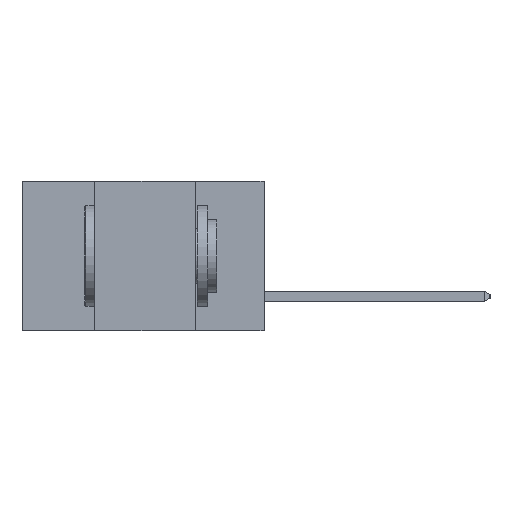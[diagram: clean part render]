
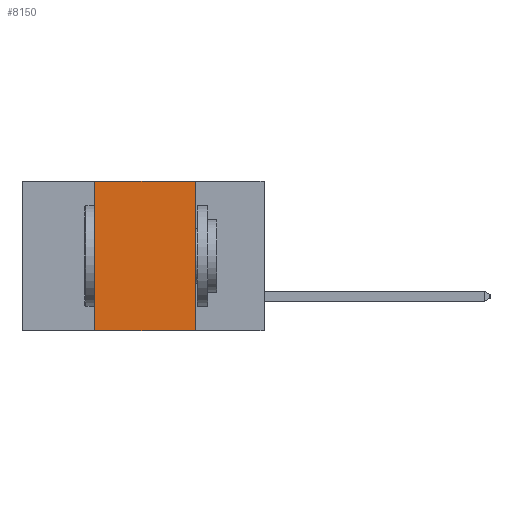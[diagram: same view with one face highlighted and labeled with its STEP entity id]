
A CAD part, left-side view. The second image highlights one B-rep face of the part: STEP entity #8150.
In plain terms, the highlighted planar face has unit normal (-1, 0, 0).
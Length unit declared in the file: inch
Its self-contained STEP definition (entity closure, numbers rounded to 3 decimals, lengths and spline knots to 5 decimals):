
#425 = EDGE_LOOP ( 'NONE', ( #8976, #8851, #8439, #8219 ) ) ;
#953 = DIRECTION ( 'NONE',  ( 0., 0., -1. ) ) ;
#1582 = VECTOR ( 'NONE', #8181, 39.37008 ) ;
#2055 = VERTEX_POINT ( 'NONE', #6297 ) ;
#2205 = EDGE_CURVE ( 'NONE', #11987, #14409, #14117, .T. ) ;
#2514 = CARTESIAN_POINT ( 'NONE',  ( 0., 0.17, -0.37 ) ) ;
#3805 = VECTOR ( 'NONE', #17910, 39.37008 ) ;
#4271 = LINE ( 'NONE', #18307, #3805 ) ;
#4373 = VECTOR ( 'NONE', #15087, 39.37008 ) ;
#6297 = CARTESIAN_POINT ( 'NONE',  ( 0., 0.17, 0. ) ) ;
#6467 = LINE ( 'NONE', #2514, #10057 ) ;
#6764 = FACE_OUTER_BOUND ( 'NONE', #425, .T. ) ;
#8150 = ADVANCED_FACE ( 'NONE', ( #6764 ), #16581, .F. ) ;
#8181 = DIRECTION ( 'NONE',  ( 0., 0., 1. ) ) ;
#8219 = ORIENTED_EDGE ( 'NONE', *, *, #12738, .T. ) ;
#8274 = CARTESIAN_POINT ( 'NONE',  ( 0., 0.42, -0.37 ) ) ;
#8325 = EDGE_CURVE ( 'NONE', #14409, #2055, #15863, .T. ) ;
#8439 = ORIENTED_EDGE ( 'NONE', *, *, #2205, .F. ) ;
#8851 = ORIENTED_EDGE ( 'NONE', *, *, #8325, .F. ) ;
#8976 = ORIENTED_EDGE ( 'NONE', *, *, #17470, .F. ) ;
#10057 = VECTOR ( 'NONE', #953, 39.37008 ) ;
#10272 = CARTESIAN_POINT ( 'NONE',  ( 0., 0.42, 0. ) ) ;
#10997 = CARTESIAN_POINT ( 'NONE',  ( 0., 0.17, -0.37 ) ) ;
#11987 = VERTEX_POINT ( 'NONE', #14861 ) ;
#12738 = EDGE_CURVE ( 'NONE', #11987, #14087, #4271, .T. ) ;
#14087 = VERTEX_POINT ( 'NONE', #10997 ) ;
#14117 = LINE ( 'NONE', #8274, #1582 ) ;
#14409 = VERTEX_POINT ( 'NONE', #10272 ) ;
#14861 = CARTESIAN_POINT ( 'NONE',  ( 0., 0.42, -0.37 ) ) ;
#15087 = DIRECTION ( 'NONE',  ( 0., -1., 0. ) ) ;
#15132 = CARTESIAN_POINT ( 'NONE',  ( 0., 0.6, 0. ) ) ;
#15863 = LINE ( 'NONE', #15132, #4373 ) ;
#16535 = DIRECTION ( 'NONE',  ( 0., 0., -1. ) ) ;
#16543 = DIRECTION ( 'NONE',  ( 1., 0., 0. ) ) ;
#16581 = PLANE ( 'NONE',  #17561 ) ;
#16584 = CARTESIAN_POINT ( 'NONE',  ( 0., 0.6, 0. ) ) ;
#17470 = EDGE_CURVE ( 'NONE', #2055, #14087, #6467, .T. ) ;
#17561 = AXIS2_PLACEMENT_3D ( 'NONE', #16584, #16543, #16535 ) ;
#17910 = DIRECTION ( 'NONE',  ( 0., -1., 0. ) ) ;
#18307 = CARTESIAN_POINT ( 'NONE',  ( 0., 0.6, -0.37 ) ) ;
